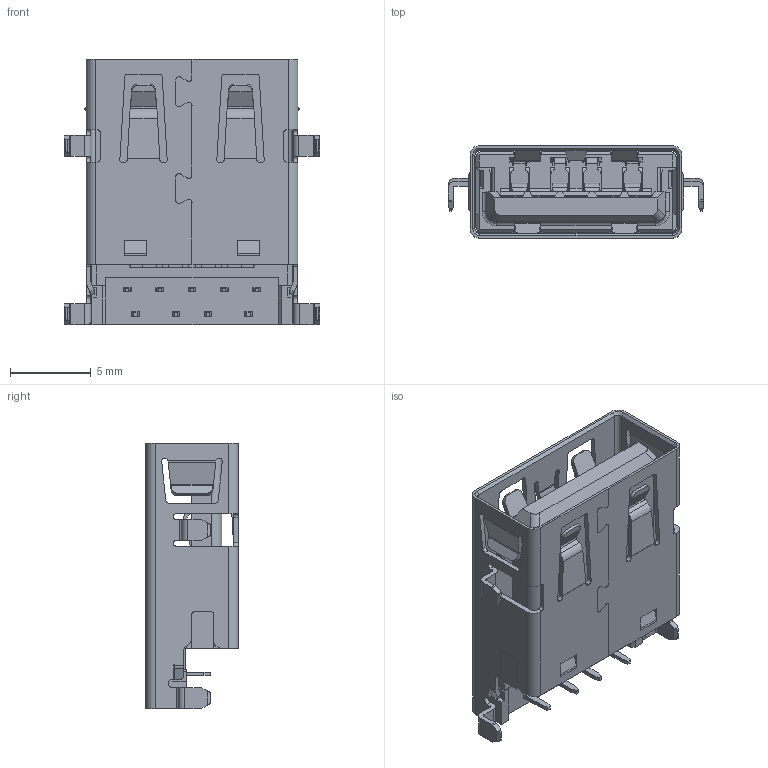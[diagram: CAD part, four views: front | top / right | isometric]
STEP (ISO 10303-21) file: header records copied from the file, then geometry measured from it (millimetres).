
FILE_DESCRIPTION (( 'STEP AP214' ), '1' );
FILE_NAME ('690H509-252-252.STEP', '2021-01-14T18:27:52', ( '' ), ( '' ), 'SwSTEP 2.0', 'SolidWorks 2020', '' );
FILE_SCHEMA (( 'AUTOMOTIVE_DESIGN' ));
Length unit declared in the file: millimetre
Products named in the file (14): Contact2 690H509-X52-252; Contact3 690H509-X52-252; Contact1 690H509-X52-252; Insulator3 690H509-X52-252; Insulator1 690H509-X52-252; Contact7 690H509-X52-252; Contact9 690H509-X52-252; Insulator2 690H509-X52-252; Contact6 690H509-X52-252; Contact4 690H509-X52-252; Contact5 690H509-X52-252; 690H509-252-252; Contact8 690H509-X52-252; Shell 690-509HX52-252
Assembly tree (13 placements, depth 2):
  690H509-252-252
    Insulator3 690H509-X52-252
    Insulator1 690H509-X52-252
    Insulator2 690H509-X52-252
    Contact1 690H509-X52-252
    Contact2 690H509-X52-252
    Contact3 690H509-X52-252
    Contact4 690H509-X52-252
    Contact5 690H509-X52-252
    Contact8 690H509-X52-252
    Contact7 690H509-X52-252
    Contact6 690H509-X52-252
    Contact9 690H509-X52-252
    Shell 690-509HX52-252
Bounding box: 15.8 x 5.72 x 16.4 mm (x, y, z)
Volume: 465.6 mm3; surface area: 2570.4 mm2
Topology: 13 solids, 13 shells, 2249 faces, 6457 edges, 4200 vertices
Faces by surface type: plane 1497, cylinder 696, bspline 40, cone 16
Entity records: 75337 total; most frequent: CARTESIAN_POINT 15475, ORIENTED_EDGE 12914, DIRECTION 11897, EDGE_CURVE 6457, VECTOR 4863, LINE 4863, VERTEX_POINT 4200, AXIS2_PLACEMENT_3D 3517
